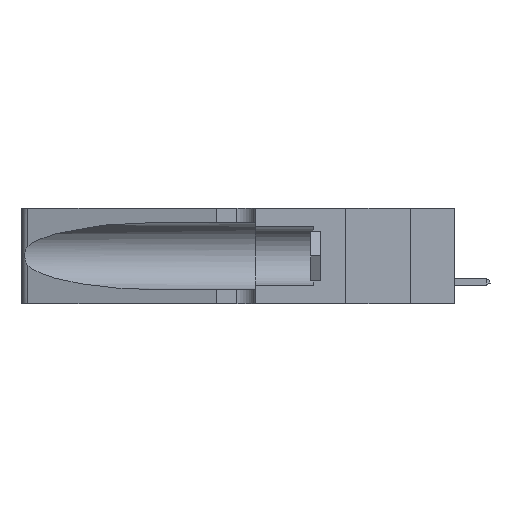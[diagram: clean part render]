
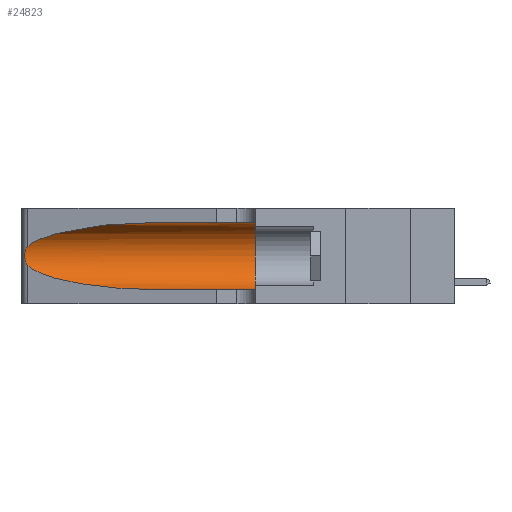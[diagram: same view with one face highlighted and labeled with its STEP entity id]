
A CAD part, left-side view. The second image highlights one B-rep face of the part: STEP entity #24823.
In plain terms, the highlighted cylindrical face has radius 3.308 mm (diameter 6.617 mm), a partial arc.
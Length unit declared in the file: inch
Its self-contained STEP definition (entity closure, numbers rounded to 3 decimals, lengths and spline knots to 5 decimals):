
#381 = CARTESIAN_POINT ( 'NONE',  ( 0.25487, 1.22718, 0.14631 ) ) ;
#497 = EDGE_CURVE ( 'NONE', #14670, #34974, #7858, .T. ) ;
#639 = DIRECTION ( 'NONE',  ( 0., -1., 0. ) ) ;
#762 = CARTESIAN_POINT ( 'NONE',  ( 0.1305, 1.61858, 0.05475 ) ) ;
#880 = CARTESIAN_POINT ( 'NONE',  ( 0.25639, 1.23186, 0.15144 ) ) ;
#1192 = CARTESIAN_POINT ( 'NONE',  ( 0.2373, 1.15595, 0.28018 ) ) ;
#1937 = ORIENTED_EDGE ( 'NONE', *, *, #35605, .T. ) ;
#3612 = CARTESIAN_POINT ( 'NONE',  ( 0.26075, 1.23896, 0.178 ) ) ;
#3668 = DIRECTION ( 'NONE',  ( 0., 1., 0. ) ) ;
#3742 = CARTESIAN_POINT ( 'NONE',  ( 0.26018, 1.23835, 0.19895 ) ) ;
#6345 = CARTESIAN_POINT ( 'NONE',  ( 0.25787, 1.23484, 0.2124 ) ) ;
#6755 = CARTESIAN_POINT ( 'NONE',  ( 0.18966, 0.96281, 0.05475 ) ) ;
#7288 = CARTESIAN_POINT ( 'NONE',  ( 0.1305, 0.72297, 0.31525 ) ) ;
#7858 = B_SPLINE_CURVE_WITH_KNOTS ( 'NONE', 3,
 ( #23454, #23325, #11715, #6345, #31727, #3742, #26448, #3612, #20702, #32226, #26315, #880, #23577, #381 ),
 .UNSPECIFIED., .F., .F.,
 ( 4, 2, 2, 2, 2, 2, 4 ),
 ( 0., 0.00027, 0.00053, 0.00107, 0.0016, 0.00187, 0.00214 ),
 .UNSPECIFIED. ) ;
#10416 = ORIENTED_EDGE ( 'NONE', *, *, #26717, .T. ) ;
#10519 = VERTEX_POINT ( 'NONE', #19125 ) ;
#10803 = VERTEX_POINT ( 'NONE', #16896 ) ;
#11078 = ORIENTED_EDGE ( 'NONE', *, *, #32560, .F. ) ;
#11419 = CARTESIAN_POINT ( 'NONE',  ( 0.1305, 0.35, 0.05475 ) ) ;
#11715 = CARTESIAN_POINT ( 'NONE',  ( 0.25639, 1.23184, 0.21858 ) ) ;
#14030 =( BOUNDED_CURVE ( )  B_SPLINE_CURVE ( 3, ( #15146, #20970, #6755, #35022 ),
 .UNSPECIFIED., .F., .T. ) 
 B_SPLINE_CURVE_WITH_KNOTS ( ( 4, 4 ),
 ( 3.44316, 4.71239 ),
 .UNSPECIFIED. ) 
 CURVE ( )  GEOMETRIC_REPRESENTATION_ITEM ( )  RATIONAL_B_SPLINE_CURVE ( ( 1., 0.87, 0.87, 1. ) ) 
 REPRESENTATION_ITEM ( '' )  );
#14670 = VERTEX_POINT ( 'NONE', #18618 ) ;
#15117 = DIRECTION ( 'NONE',  ( 0., -1., 0. ) ) ;
#15146 = CARTESIAN_POINT ( 'NONE',  ( 0.25487, 1.22718, 0.14631 ) ) ;
#15288 = VECTOR ( 'NONE', #639, 39.37008 ) ;
#15817 = FACE_OUTER_BOUND ( 'NONE', #32557, .T. ) ;
#15893 = VECTOR ( 'NONE', #35731, 39.37008 ) ;
#16215 = AXIS2_PLACEMENT_3D ( 'NONE', #23962, #15117, #26830 ) ;
#16896 = CARTESIAN_POINT ( 'NONE',  ( 0.1305, 0.72297, 0.31525 ) ) ;
#18237 = CARTESIAN_POINT ( 'NONE',  ( 0.1305, 1.61858, 0.31525 ) ) ;
#18618 = CARTESIAN_POINT ( 'NONE',  ( 0.25487, 1.22718, 0.22369 ) ) ;
#19125 = CARTESIAN_POINT ( 'NONE',  ( 0.1305, 0.35, 0.31525 ) ) ;
#19148 = ORIENTED_EDGE ( 'NONE', *, *, #33626, .F. ) ;
#19291 = ORIENTED_EDGE ( 'NONE', *, *, #21537, .T. ) ;
#20256 = CIRCLE ( 'NONE', #24960, 0.13025 ) ;
#20702 = CARTESIAN_POINT ( 'NONE',  ( 0.26017, 1.23833, 0.17102 ) ) ;
#20970 = CARTESIAN_POINT ( 'NONE',  ( 0.2373, 1.15595, 0.08982 ) ) ;
#21124 = CARTESIAN_POINT ( 'NONE',  ( 0.1305, 0.72297, 0.05475 ) ) ;
#21147 = CARTESIAN_POINT ( 'NONE',  ( 0.25487, 1.22718, 0.22369 ) ) ;
#21537 = EDGE_CURVE ( 'NONE', #10803, #14670, #30057, .T. ) ;
#22872 = LINE ( 'NONE', #762, #15288 ) ;
#23137 = CARTESIAN_POINT ( 'NONE',  ( 0.1305, 0.35, 0.185 ) ) ;
#23233 = ORIENTED_EDGE ( 'NONE', *, *, #497, .T. ) ;
#23325 = CARTESIAN_POINT ( 'NONE',  ( 0.25555, 1.22994, 0.2215 ) ) ;
#23392 = CARTESIAN_POINT ( 'NONE',  ( 0.25487, 1.22718, 0.14631 ) ) ;
#23402 = CYLINDRICAL_SURFACE ( 'NONE', #16215, 0.13025 ) ;
#23454 = CARTESIAN_POINT ( 'NONE',  ( 0.25487, 1.22718, 0.22369 ) ) ;
#23577 = CARTESIAN_POINT ( 'NONE',  ( 0.25555, 1.22993, 0.14849 ) ) ;
#23627 = DIRECTION ( 'NONE',  ( 0., 0., 1. ) ) ;
#23962 = CARTESIAN_POINT ( 'NONE',  ( 0.1305, 1.61858, 0.185 ) ) ;
#24823 = ADVANCED_FACE ( 'NONE', ( #15817 ), #23402, .F. ) ;
#24960 = AXIS2_PLACEMENT_3D ( 'NONE', #23137, #3668, #23627 ) ;
#26315 = CARTESIAN_POINT ( 'NONE',  ( 0.25789, 1.23486, 0.15765 ) ) ;
#26448 = CARTESIAN_POINT ( 'NONE',  ( 0.26075, 1.23896, 0.19203 ) ) ;
#26717 = EDGE_CURVE ( 'NONE', #31704, #29546, #22872, .T. ) ;
#26830 = DIRECTION ( 'NONE',  ( 0., 0., -1. ) ) ;
#29546 = VERTEX_POINT ( 'NONE', #11419 ) ;
#30057 =( BOUNDED_CURVE ( )  B_SPLINE_CURVE ( 3, ( #7288, #32551, #1192, #21147 ),
 .UNSPECIFIED., .F., .F. ) 
 B_SPLINE_CURVE_WITH_KNOTS ( ( 4, 4 ),
 ( 1.5708, 2.84003 ),
 .UNSPECIFIED. ) 
 CURVE ( )  GEOMETRIC_REPRESENTATION_ITEM ( )  RATIONAL_B_SPLINE_CURVE ( ( 1., 0.87, 0.87, 1. ) ) 
 REPRESENTATION_ITEM ( '' )  );
#31704 = VERTEX_POINT ( 'NONE', #21124 ) ;
#31727 = CARTESIAN_POINT ( 'NONE',  ( 0.25854, 1.2359, 0.20912 ) ) ;
#32226 = CARTESIAN_POINT ( 'NONE',  ( 0.25856, 1.23593, 0.16098 ) ) ;
#32551 = CARTESIAN_POINT ( 'NONE',  ( 0.18966, 0.96281, 0.31525 ) ) ;
#32557 = EDGE_LOOP ( 'NONE', ( #19291, #23233, #1937, #10416, #19148, #11078 ) ) ;
#32560 = EDGE_CURVE ( 'NONE', #10803, #10519, #33348, .T. ) ;
#33348 = LINE ( 'NONE', #18237, #15893 ) ;
#33626 = EDGE_CURVE ( 'NONE', #10519, #29546, #20256, .T. ) ;
#34974 = VERTEX_POINT ( 'NONE', #23392 ) ;
#35022 = CARTESIAN_POINT ( 'NONE',  ( 0.1305, 0.72297, 0.05475 ) ) ;
#35605 = EDGE_CURVE ( 'NONE', #34974, #31704, #14030, .T. ) ;
#35731 = DIRECTION ( 'NONE',  ( 0., -1., 0. ) ) ;
